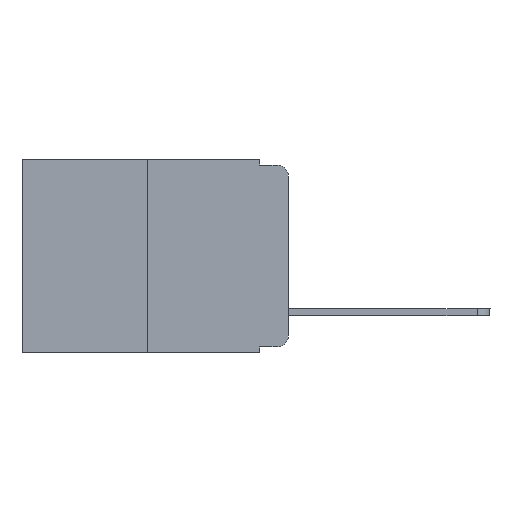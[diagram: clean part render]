
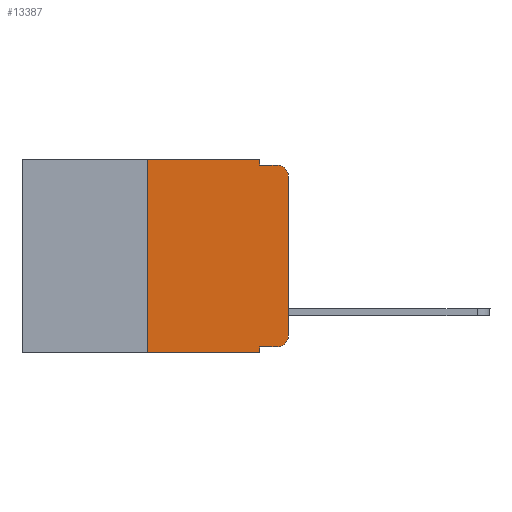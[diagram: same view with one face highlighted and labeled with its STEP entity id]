
A CAD part, left-side view. The second image highlights one B-rep face of the part: STEP entity #13387.
In plain terms, the highlighted planar face has unit normal (-1, 0, 0).
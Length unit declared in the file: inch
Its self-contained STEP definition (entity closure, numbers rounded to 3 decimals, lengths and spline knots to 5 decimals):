
#377 = EDGE_CURVE ( 'NONE', #7959, #16637, #10708, .T. ) ;
#671 = DIRECTION ( 'NONE',  ( 0., -1., 0. ) ) ;
#692 = CARTESIAN_POINT ( 'NONE',  ( 0., 0.051, -0.01 ) ) ;
#1080 = CARTESIAN_POINT ( 'NONE',  ( 0., 0., 0. ) ) ;
#1158 = CARTESIAN_POINT ( 'NONE',  ( 0., 0., -0.03 ) ) ;
#1503 = VERTEX_POINT ( 'NONE', #4878 ) ;
#1650 = CARTESIAN_POINT ( 'NONE',  ( 0., 0.25, -0.343 ) ) ;
#1926 = LINE ( 'NONE', #19983, #12567 ) ;
#2001 = VERTEX_POINT ( 'NONE', #1158 ) ;
#2060 = CARTESIAN_POINT ( 'NONE',  ( 0., 0.051, -0.333 ) ) ;
#2103 = VECTOR ( 'NONE', #20427, 39.37008 ) ;
#2587 = CARTESIAN_POINT ( 'NONE',  ( 0., 0.473, 0. ) ) ;
#2955 = DIRECTION ( 'NONE',  ( 0., 0., -1. ) ) ;
#3599 = ORIENTED_EDGE ( 'NONE', *, *, #377, .F. ) ;
#3630 = VECTOR ( 'NONE', #13591, 39.37008 ) ;
#3880 = CARTESIAN_POINT ( 'NONE',  ( 0., 0.473, 0. ) ) ;
#4060 = EDGE_CURVE ( 'NONE', #19253, #14486, #1926, .T. ) ;
#4188 = EDGE_CURVE ( 'NONE', #2001, #15626, #11026, .T. ) ;
#4282 = CARTESIAN_POINT ( 'NONE',  ( 0., 0.02, -0.03 ) ) ;
#4653 = CARTESIAN_POINT ( 'NONE',  ( 0., 0.051, -0.333 ) ) ;
#4726 = ORIENTED_EDGE ( 'NONE', *, *, #5111, .T. ) ;
#4878 = CARTESIAN_POINT ( 'NONE',  ( 0., 0.25, 0. ) ) ;
#5111 = EDGE_CURVE ( 'NONE', #16873, #11094, #7217, .T. ) ;
#5397 = EDGE_CURVE ( 'NONE', #7959, #16873, #11496, .T. ) ;
#5954 = ORIENTED_EDGE ( 'NONE', *, *, #4060, .F. ) ;
#6350 = EDGE_CURVE ( 'NONE', #13684, #1503, #15429, .T. ) ;
#6690 = CARTESIAN_POINT ( 'NONE',  ( 0., 0.051, 0. ) ) ;
#7063 = ORIENTED_EDGE ( 'NONE', *, *, #19373, .F. ) ;
#7209 = VECTOR ( 'NONE', #14418, 39.37008 ) ;
#7217 = CIRCLE ( 'NONE', #11568, 0.02 ) ;
#7959 = VERTEX_POINT ( 'NONE', #2060 ) ;
#8748 = DIRECTION ( 'NONE',  ( 0., -1., 0. ) ) ;
#8884 = DIRECTION ( 'NONE',  ( 1., 0., 0. ) ) ;
#9133 = LINE ( 'NONE', #12148, #18261 ) ;
#10047 = CARTESIAN_POINT ( 'NONE',  ( 0., 0.25, 0. ) ) ;
#10185 = CARTESIAN_POINT ( 'NONE',  ( 0., 0.051, 0. ) ) ;
#10708 = LINE ( 'NONE', #10185, #3630 ) ;
#11026 = CIRCLE ( 'NONE', #18617, 0.02 ) ;
#11094 = VERTEX_POINT ( 'NONE', #17227 ) ;
#11336 = CARTESIAN_POINT ( 'NONE',  ( 0., 0.051, -0.01 ) ) ;
#11496 = LINE ( 'NONE', #4653, #7209 ) ;
#11568 = AXIS2_PLACEMENT_3D ( 'NONE', #12653, #15991, #2955 ) ;
#11989 = PLANE ( 'NONE',  #16884 ) ;
#12148 = CARTESIAN_POINT ( 'NONE',  ( 0., 0.473, -0.343 ) ) ;
#12567 = VECTOR ( 'NONE', #18397, 39.37008 ) ;
#12653 = CARTESIAN_POINT ( 'NONE',  ( 0., 0.02, -0.313 ) ) ;
#13227 = CARTESIAN_POINT ( 'NONE',  ( 0., 0.02, -0.01 ) ) ;
#13387 = ADVANCED_FACE ( 'NONE', ( #16599 ), #11989, .F. ) ;
#13591 = DIRECTION ( 'NONE',  ( 0., 0., -1. ) ) ;
#13652 = VECTOR ( 'NONE', #16502, 39.37008 ) ;
#13684 = VERTEX_POINT ( 'NONE', #1650 ) ;
#13858 = ORIENTED_EDGE ( 'NONE', *, *, #4188, .T. ) ;
#14418 = DIRECTION ( 'NONE',  ( 0., -1., 0. ) ) ;
#14486 = VERTEX_POINT ( 'NONE', #692 ) ;
#14589 = ORIENTED_EDGE ( 'NONE', *, *, #20190, .T. ) ;
#15222 = ORIENTED_EDGE ( 'NONE', *, *, #6350, .F. ) ;
#15429 = LINE ( 'NONE', #10047, #13652 ) ;
#15589 = VECTOR ( 'NONE', #8748, 39.37008 ) ;
#15626 = VERTEX_POINT ( 'NONE', #13227 ) ;
#15813 = VECTOR ( 'NONE', #17997, 39.37008 ) ;
#15854 = ORIENTED_EDGE ( 'NONE', *, *, #19851, .F. ) ;
#15985 = EDGE_CURVE ( 'NONE', #13684, #16637, #9133, .T. ) ;
#15991 = DIRECTION ( 'NONE',  ( -1., 0., 0. ) ) ;
#16052 = LINE ( 'NONE', #11336, #15813 ) ;
#16293 = LINE ( 'NONE', #1080, #2103 ) ;
#16358 = ORIENTED_EDGE ( 'NONE', *, *, #5397, .T. ) ;
#16502 = DIRECTION ( 'NONE',  ( 0., 0., 1. ) ) ;
#16599 = FACE_OUTER_BOUND ( 'NONE', #18022, .T. ) ;
#16637 = VERTEX_POINT ( 'NONE', #18623 ) ;
#16842 = ORIENTED_EDGE ( 'NONE', *, *, #15985, .T. ) ;
#16873 = VERTEX_POINT ( 'NONE', #17692 ) ;
#16884 = AXIS2_PLACEMENT_3D ( 'NONE', #2587, #8884, #20232 ) ;
#16947 = DIRECTION ( 'NONE',  ( -1., 0., 0. ) ) ;
#17150 = DIRECTION ( 'NONE',  ( 0., 0., -1. ) ) ;
#17227 = CARTESIAN_POINT ( 'NONE',  ( 0., 0., -0.313 ) ) ;
#17692 = CARTESIAN_POINT ( 'NONE',  ( 0., 0.02, -0.333 ) ) ;
#17997 = DIRECTION ( 'NONE',  ( 0., -1., 0. ) ) ;
#18022 = EDGE_LOOP ( 'NONE', ( #14589, #13858, #15854, #5954, #7063, #15222, #16842, #3599, #16358, #4726 ) ) ;
#18261 = VECTOR ( 'NONE', #671, 39.37008 ) ;
#18397 = DIRECTION ( 'NONE',  ( 0., 0., -1. ) ) ;
#18617 = AXIS2_PLACEMENT_3D ( 'NONE', #4282, #16947, #17150 ) ;
#18623 = CARTESIAN_POINT ( 'NONE',  ( 0., 0.051, -0.343 ) ) ;
#19253 = VERTEX_POINT ( 'NONE', #6690 ) ;
#19373 = EDGE_CURVE ( 'NONE', #1503, #19253, #20407, .T. ) ;
#19851 = EDGE_CURVE ( 'NONE', #14486, #15626, #16052, .T. ) ;
#19983 = CARTESIAN_POINT ( 'NONE',  ( 0., 0.051, 0. ) ) ;
#20190 = EDGE_CURVE ( 'NONE', #11094, #2001, #16293, .T. ) ;
#20232 = DIRECTION ( 'NONE',  ( 0., 0., -1. ) ) ;
#20407 = LINE ( 'NONE', #3880, #15589 ) ;
#20427 = DIRECTION ( 'NONE',  ( 0., 0., 1. ) ) ;
